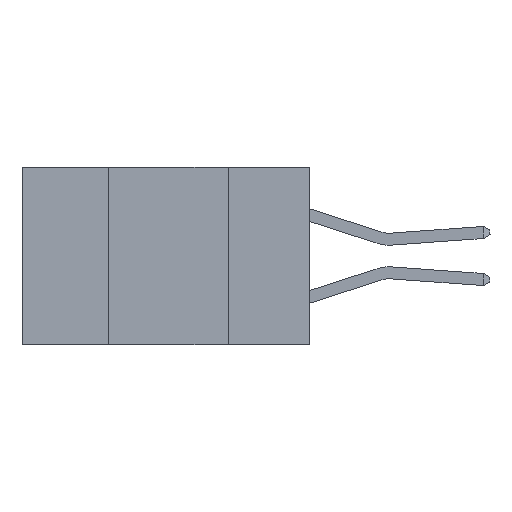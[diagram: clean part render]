
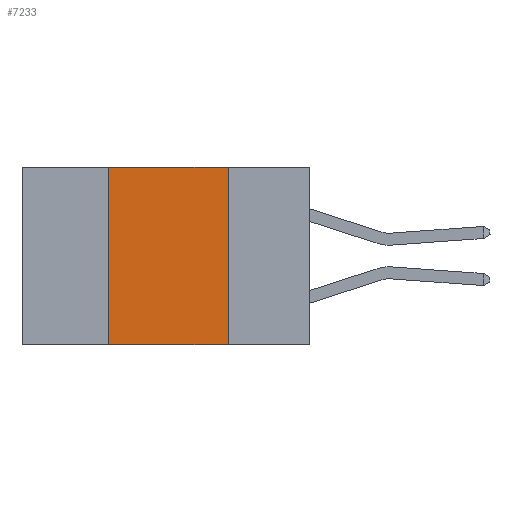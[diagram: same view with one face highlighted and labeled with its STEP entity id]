
A CAD part, left-side view. The second image highlights one B-rep face of the part: STEP entity #7233.
In plain terms, the highlighted planar face has unit normal (-1, 0, 0).
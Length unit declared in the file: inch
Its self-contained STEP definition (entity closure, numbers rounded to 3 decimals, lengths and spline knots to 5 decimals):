
#1326 = VECTOR ( 'NONE', #18782, 39.37008 ) ;
#2168 = LINE ( 'NONE', #23881, #12339 ) ;
#2897 = DIRECTION ( 'NONE',  ( 1., 0., 0. ) ) ;
#3035 = VERTEX_POINT ( 'NONE', #12533 ) ;
#3239 = AXIS2_PLACEMENT_3D ( 'NONE', #15106, #2897, #17168 ) ;
#4023 = ORIENTED_EDGE ( 'NONE', *, *, #12535, .F. ) ;
#5125 = ORIENTED_EDGE ( 'NONE', *, *, #24608, .F. ) ;
#5231 = EDGE_CURVE ( 'NONE', #7882, #24787, #25955, .T. ) ;
#7233 = ADVANCED_FACE ( 'NONE', ( #13512 ), #23130, .F. ) ;
#7380 = LINE ( 'NONE', #16698, #1326 ) ;
#7882 = VERTEX_POINT ( 'NONE', #26094 ) ;
#9741 = VECTOR ( 'NONE', #22195, 39.37008 ) ;
#10082 = ORIENTED_EDGE ( 'NONE', *, *, #19319, .F. ) ;
#11056 = LINE ( 'NONE', #20235, #9741 ) ;
#12339 = VECTOR ( 'NONE', #25879, 39.37008 ) ;
#12533 = CARTESIAN_POINT ( 'NONE',  ( 0., 0.17, 0. ) ) ;
#12535 = EDGE_CURVE ( 'NONE', #17807, #3035, #11056, .T. ) ;
#13004 = CARTESIAN_POINT ( 'NONE',  ( 0., 0.42, 0. ) ) ;
#13512 = FACE_OUTER_BOUND ( 'NONE', #18438, .T. ) ;
#15106 = CARTESIAN_POINT ( 'NONE',  ( 0., 0.6, 0. ) ) ;
#16698 = CARTESIAN_POINT ( 'NONE',  ( 0., 0.17, 0. ) ) ;
#17168 = DIRECTION ( 'NONE',  ( 0., 0., -1. ) ) ;
#17235 = CARTESIAN_POINT ( 'NONE',  ( 0., 0.17, -0.37 ) ) ;
#17807 = VERTEX_POINT ( 'NONE', #13004 ) ;
#18438 = EDGE_LOOP ( 'NONE', ( #5125, #4023, #10082, #24665 ) ) ;
#18782 = DIRECTION ( 'NONE',  ( 0., 0., -1. ) ) ;
#19319 = EDGE_CURVE ( 'NONE', #7882, #17807, #2168, .T. ) ;
#20235 = CARTESIAN_POINT ( 'NONE',  ( 0., 0.6, 0. ) ) ;
#20701 = VECTOR ( 'NONE', #25144, 39.37008 ) ;
#21158 = CARTESIAN_POINT ( 'NONE',  ( 0., 0.6, -0.37 ) ) ;
#22195 = DIRECTION ( 'NONE',  ( 0., -1., 0. ) ) ;
#23130 = PLANE ( 'NONE',  #3239 ) ;
#23881 = CARTESIAN_POINT ( 'NONE',  ( 0., 0.42, 0. ) ) ;
#24608 = EDGE_CURVE ( 'NONE', #3035, #24787, #7380, .T. ) ;
#24665 = ORIENTED_EDGE ( 'NONE', *, *, #5231, .T. ) ;
#24787 = VERTEX_POINT ( 'NONE', #17235 ) ;
#25144 = DIRECTION ( 'NONE',  ( 0., -1., 0. ) ) ;
#25879 = DIRECTION ( 'NONE',  ( 0., 0., 1. ) ) ;
#25955 = LINE ( 'NONE', #21158, #20701 ) ;
#26094 = CARTESIAN_POINT ( 'NONE',  ( 0., 0.42, -0.37 ) ) ;
